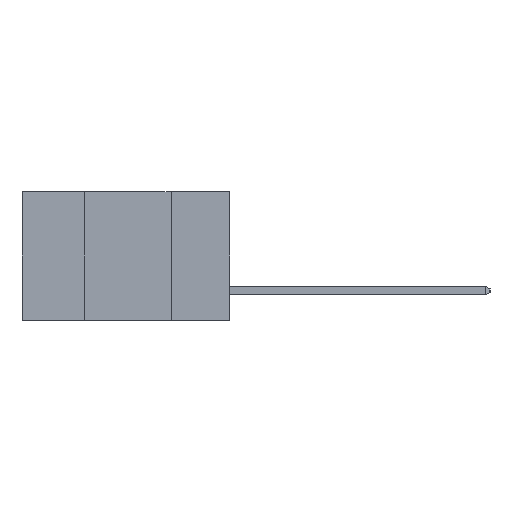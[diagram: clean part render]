
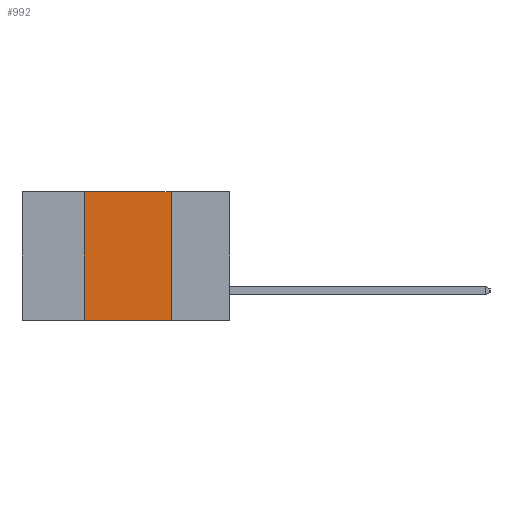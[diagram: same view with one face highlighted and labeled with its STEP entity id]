
A CAD part, left-side view. The second image highlights one B-rep face of the part: STEP entity #992.
In plain terms, the highlighted planar face has unit normal (-1, 0, 0).
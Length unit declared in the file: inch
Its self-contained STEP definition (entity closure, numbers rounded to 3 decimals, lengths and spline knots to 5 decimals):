
#47 = VECTOR ( 'NONE', #10341, 39.37008 ) ;
#222 = EDGE_CURVE ( 'NONE', #2504, #7090, #1556, .T. ) ;
#354 = AXIS2_PLACEMENT_3D ( 'NONE', #9413, #8726, #8714 ) ;
#825 = VECTOR ( 'NONE', #4341, 39.37008 ) ;
#887 = EDGE_CURVE ( 'NONE', #2504, #3925, #4445, .T. ) ;
#992 = ADVANCED_FACE ( 'NONE', ( #8938 ), #10410, .F. ) ;
#1467 = EDGE_CURVE ( 'NONE', #3925, #5709, #7260, .T. ) ;
#1506 = EDGE_LOOP ( 'NONE', ( #6722, #2703, #4541, #4770 ) ) ;
#1556 = LINE ( 'NONE', #10205, #3805 ) ;
#2065 = EDGE_CURVE ( 'NONE', #5709, #7090, #3381, .T. ) ;
#2323 = CARTESIAN_POINT ( 'NONE',  ( 0., 0.42, -0.37 ) ) ;
#2391 = CARTESIAN_POINT ( 'NONE',  ( 0., 0.42, 0. ) ) ;
#2504 = VERTEX_POINT ( 'NONE', #2323 ) ;
#2703 = ORIENTED_EDGE ( 'NONE', *, *, #1467, .F. ) ;
#3381 = LINE ( 'NONE', #3796, #825 ) ;
#3796 = CARTESIAN_POINT ( 'NONE',  ( 0., 0.17, -0.37 ) ) ;
#3805 = VECTOR ( 'NONE', #5851, 39.37008 ) ;
#3925 = VERTEX_POINT ( 'NONE', #2391 ) ;
#4267 = CARTESIAN_POINT ( 'NONE',  ( 0., 0.17, -0.37 ) ) ;
#4341 = DIRECTION ( 'NONE',  ( 0., 0., -1. ) ) ;
#4445 = LINE ( 'NONE', #6297, #47 ) ;
#4541 = ORIENTED_EDGE ( 'NONE', *, *, #887, .F. ) ;
#4770 = ORIENTED_EDGE ( 'NONE', *, *, #222, .T. ) ;
#5709 = VERTEX_POINT ( 'NONE', #9326 ) ;
#5851 = DIRECTION ( 'NONE',  ( 0., -1., 0. ) ) ;
#6297 = CARTESIAN_POINT ( 'NONE',  ( 0., 0.42, -0.37 ) ) ;
#6722 = ORIENTED_EDGE ( 'NONE', *, *, #2065, .F. ) ;
#7090 = VERTEX_POINT ( 'NONE', #4267 ) ;
#7098 = CARTESIAN_POINT ( 'NONE',  ( 0., 0.6, 0. ) ) ;
#7208 = DIRECTION ( 'NONE',  ( 0., -1., 0. ) ) ;
#7260 = LINE ( 'NONE', #7098, #9037 ) ;
#8714 = DIRECTION ( 'NONE',  ( 0., 0., -1. ) ) ;
#8726 = DIRECTION ( 'NONE',  ( 1., 0., 0. ) ) ;
#8938 = FACE_OUTER_BOUND ( 'NONE', #1506, .T. ) ;
#9037 = VECTOR ( 'NONE', #7208, 39.37008 ) ;
#9326 = CARTESIAN_POINT ( 'NONE',  ( 0., 0.17, 0. ) ) ;
#9413 = CARTESIAN_POINT ( 'NONE',  ( 0., 0.6, 0. ) ) ;
#10205 = CARTESIAN_POINT ( 'NONE',  ( 0., 0.6, -0.37 ) ) ;
#10341 = DIRECTION ( 'NONE',  ( 0., 0., 1. ) ) ;
#10410 = PLANE ( 'NONE',  #354 ) ;
